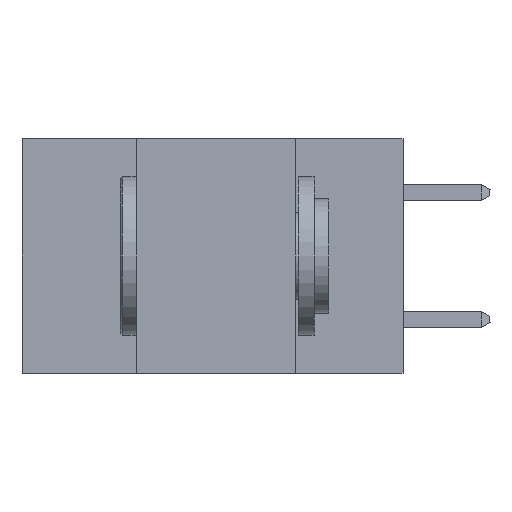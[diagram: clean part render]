
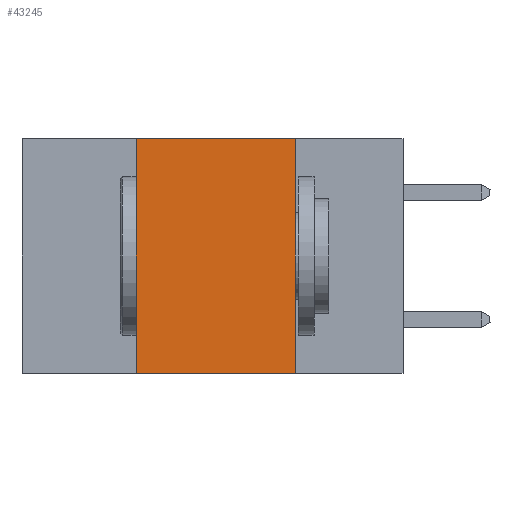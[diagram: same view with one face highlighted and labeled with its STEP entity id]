
A CAD part, left-side view. The second image highlights one B-rep face of the part: STEP entity #43245.
In plain terms, the highlighted planar face has unit normal (-1, 0, 0).
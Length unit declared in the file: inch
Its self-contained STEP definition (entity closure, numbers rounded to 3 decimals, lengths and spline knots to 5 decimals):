
#1197 = CARTESIAN_POINT ( 'NONE',  ( 0., 0.17, 0. ) ) ;
#3156 = VECTOR ( 'NONE', #10269, 39.37008 ) ;
#3652 = EDGE_CURVE ( 'NONE', #18379, #14040, #4259, .T. ) ;
#4026 = CARTESIAN_POINT ( 'NONE',  ( 0., 0.42, -0.37 ) ) ;
#4259 = LINE ( 'NONE', #17492, #3156 ) ;
#4623 = PLANE ( 'NONE',  #11604 ) ;
#5869 = CARTESIAN_POINT ( 'NONE',  ( 0., 0.17, 0. ) ) ;
#6948 = ORIENTED_EDGE ( 'NONE', *, *, #33133, .T. ) ;
#8174 = DIRECTION ( 'NONE',  ( 1., 0., 0. ) ) ;
#9197 = VERTEX_POINT ( 'NONE', #36985 ) ;
#10269 = DIRECTION ( 'NONE',  ( 0., 0., 1. ) ) ;
#11604 = AXIS2_PLACEMENT_3D ( 'NONE', #40216, #8174, #33250 ) ;
#11799 = VECTOR ( 'NONE', #34400, 39.37008 ) ;
#12933 = LINE ( 'NONE', #30703, #11799 ) ;
#14040 = VERTEX_POINT ( 'NONE', #45670 ) ;
#17148 = VERTEX_POINT ( 'NONE', #1197 ) ;
#17492 = CARTESIAN_POINT ( 'NONE',  ( 0., 0.42, 0. ) ) ;
#18141 = LINE ( 'NONE', #5869, #45416 ) ;
#18379 = VERTEX_POINT ( 'NONE', #4026 ) ;
#21860 = DIRECTION ( 'NONE',  ( 0., -1., 0. ) ) ;
#22581 = VECTOR ( 'NONE', #21860, 39.37008 ) ;
#24421 = ORIENTED_EDGE ( 'NONE', *, *, #36369, .F. ) ;
#28780 = EDGE_LOOP ( 'NONE', ( #24421, #44451, #46019, #6948 ) ) ;
#30258 = FACE_OUTER_BOUND ( 'NONE', #28780, .T. ) ;
#30703 = CARTESIAN_POINT ( 'NONE',  ( 0., 0.6, 0. ) ) ;
#33133 = EDGE_CURVE ( 'NONE', #18379, #9197, #33210, .T. ) ;
#33210 = LINE ( 'NONE', #36070, #22581 ) ;
#33250 = DIRECTION ( 'NONE',  ( 0., 0., -1. ) ) ;
#34400 = DIRECTION ( 'NONE',  ( 0., -1., 0. ) ) ;
#36070 = CARTESIAN_POINT ( 'NONE',  ( 0., 0.6, -0.37 ) ) ;
#36369 = EDGE_CURVE ( 'NONE', #17148, #9197, #18141, .T. ) ;
#36985 = CARTESIAN_POINT ( 'NONE',  ( 0., 0.17, -0.37 ) ) ;
#38769 = EDGE_CURVE ( 'NONE', #14040, #17148, #12933, .T. ) ;
#40216 = CARTESIAN_POINT ( 'NONE',  ( 0., 0.6, 0. ) ) ;
#43245 = ADVANCED_FACE ( 'NONE', ( #30258 ), #4623, .F. ) ;
#44451 = ORIENTED_EDGE ( 'NONE', *, *, #38769, .F. ) ;
#44817 = DIRECTION ( 'NONE',  ( 0., 0., -1. ) ) ;
#45416 = VECTOR ( 'NONE', #44817, 39.37008 ) ;
#45670 = CARTESIAN_POINT ( 'NONE',  ( 0., 0.42, 0. ) ) ;
#46019 = ORIENTED_EDGE ( 'NONE', *, *, #3652, .F. ) ;
